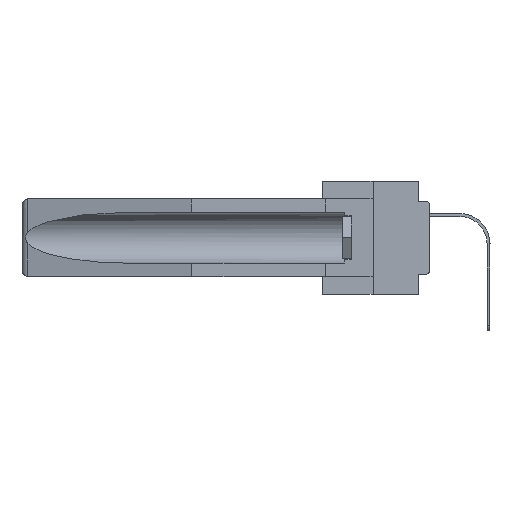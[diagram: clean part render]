
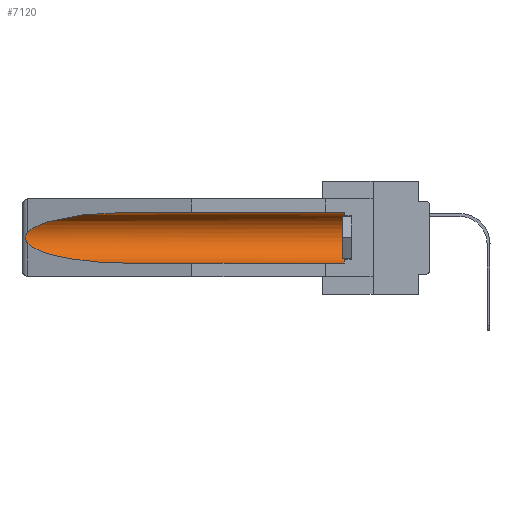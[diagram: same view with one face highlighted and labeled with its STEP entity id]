
A CAD part, left-side view. The second image highlights one B-rep face of the part: STEP entity #7120.
In plain terms, the highlighted cylindrical face has radius 2.857 mm (diameter 5.715 mm), a partial arc.
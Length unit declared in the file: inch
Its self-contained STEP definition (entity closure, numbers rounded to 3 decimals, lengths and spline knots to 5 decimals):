
#655 = ORIENTED_EDGE ( 'NONE', *, *, #25167, .F. ) ;
#1050 = CARTESIAN_POINT ( 'NONE',  ( 0.155, -0.30754, -0.284 ) ) ;
#1135 = ORIENTED_EDGE ( 'NONE', *, *, #18949, .T. ) ;
#1339 = LINE ( 'NONE', #1050, #6157 ) ;
#2214 = CARTESIAN_POINT ( 'NONE',  ( 0.26537, 1.52718, -0.19328 ) ) ;
#2487 = CARTESIAN_POINT ( 'NONE',  ( 0.26537, 1.52718, -0.19328 ) ) ;
#3384 = VERTEX_POINT ( 'NONE', #7157 ) ;
#4302 = CARTESIAN_POINT ( 'NONE',  ( 0.155, 1.07973, -0.284 ) ) ;
#4368 =( BOUNDED_CURVE ( )  B_SPLINE_CURVE ( 3, ( #22497, #22637, #20233, #8816 ),
 .UNSPECIFIED., .F., .F. ) 
 B_SPLINE_CURVE_WITH_KNOTS ( ( 4, 4 ),
 ( 4.71239, 6.08839 ),
 .UNSPECIFIED. ) 
 CURVE ( )  GEOMETRIC_REPRESENTATION_ITEM ( )  RATIONAL_B_SPLINE_CURVE ( ( 1., 0.848, 0.848, 1. ) ) 
 REPRESENTATION_ITEM ( '' )  );
#4454 = CARTESIAN_POINT ( 'NONE',  ( 0.26654, 1.53092, -0.15636 ) ) ;
#5358 = DIRECTION ( 'NONE',  ( 0., -1., 0. ) ) ;
#5659 = DIRECTION ( 'NONE',  ( 0., 0., 1. ) ) ;
#5753 = CARTESIAN_POINT ( 'NONE',  ( 0.25451, 1.48313, -0.24835 ) ) ;
#6157 = VECTOR ( 'NONE', #10702, 39.37008 ) ;
#6313 = CIRCLE ( 'NONE', #12603, 0.1125 ) ;
#6398 = CARTESIAN_POINT ( 'NONE',  ( 0.26537, 1.52718, -0.14972 ) ) ;
#6467 = VERTEX_POINT ( 'NONE', #2214 ) ;
#7002 = CARTESIAN_POINT ( 'NONE',  ( 0.26597, 1.52961, -0.15275 ) ) ;
#7120 = ADVANCED_FACE ( 'NONE', ( #10876 ), #11166, .F. ) ;
#7157 = CARTESIAN_POINT ( 'NONE',  ( 0.155, 1.07973, -0.059 ) ) ;
#7757 = EDGE_CURVE ( 'NONE', #17852, #29393, #6313, .T. ) ;
#8816 = CARTESIAN_POINT ( 'NONE',  ( 0.26537, 1.52718, -0.14972 ) ) ;
#9173 = VERTEX_POINT ( 'NONE', #6398 ) ;
#9777 = VERTEX_POINT ( 'NONE', #4302 ) ;
#10536 = EDGE_CURVE ( 'NONE', #29393, #3384, #24402, .T. ) ;
#10702 = DIRECTION ( 'NONE',  ( 0., 1., 0. ) ) ;
#10876 = FACE_OUTER_BOUND ( 'NONE', #13309, .T. ) ;
#11166 = CYLINDRICAL_SURFACE ( 'NONE', #19737, 0.1125 ) ;
#11267 = CARTESIAN_POINT ( 'NONE',  ( 0.26597, 1.5296, -0.19026 ) ) ;
#11540 = CARTESIAN_POINT ( 'NONE',  ( 0.2673, 1.5327, -0.16383 ) ) ;
#12603 = AXIS2_PLACEMENT_3D ( 'NONE', #19378, #5358, #5659 ) ;
#12727 = CARTESIAN_POINT ( 'NONE',  ( 0.21114, 1.30732, -0.284 ) ) ;
#12954 = CARTESIAN_POINT ( 'NONE',  ( 0.155, -0.30754, -0.059 ) ) ;
#13109 = B_SPLINE_CURVE_WITH_KNOTS ( 'NONE', 3,
 ( #18622, #7002, #4454, #11540, #18177, #23108, #27356, #29472, #11267, #2487 ),
 .UNSPECIFIED., .F., .F.,
 ( 4, 2, 2, 2, 4 ),
 ( 0., 0.00029, 0.00058, 0.00087, 0.00117 ),
 .UNSPECIFIED. ) ;
#13309 = EDGE_LOOP ( 'NONE', ( #1135, #24173, #13916, #655, #18756, #29010 ) ) ;
#13916 = ORIENTED_EDGE ( 'NONE', *, *, #20486, .T. ) ;
#17683 = CARTESIAN_POINT ( 'NONE',  ( 0.26537, 1.52718, -0.19328 ) ) ;
#17852 = VERTEX_POINT ( 'NONE', #20982 ) ;
#18177 = CARTESIAN_POINT ( 'NONE',  ( 0.2675, 1.53308, -0.16763 ) ) ;
#18622 = CARTESIAN_POINT ( 'NONE',  ( 0.26537, 1.52718, -0.14972 ) ) ;
#18756 = ORIENTED_EDGE ( 'NONE', *, *, #7757, .T. ) ;
#18949 = EDGE_CURVE ( 'NONE', #3384, #9173, #4368, .T. ) ;
#19170 = CARTESIAN_POINT ( 'NONE',  ( 0.155, 0.126, -0.059 ) ) ;
#19378 = CARTESIAN_POINT ( 'NONE',  ( 0.155, 0.126, -0.1715 ) ) ;
#19421 = VECTOR ( 'NONE', #22117, 39.37008 ) ;
#19737 = AXIS2_PLACEMENT_3D ( 'NONE', #20333, #29091, #26829 ) ;
#20233 = CARTESIAN_POINT ( 'NONE',  ( 0.25451, 1.48313, -0.09465 ) ) ;
#20333 = CARTESIAN_POINT ( 'NONE',  ( 0.155, -0.30754, -0.1715 ) ) ;
#20486 = EDGE_CURVE ( 'NONE', #6467, #9777, #24182, .T. ) ;
#20982 = CARTESIAN_POINT ( 'NONE',  ( 0.155, 0.126, -0.284 ) ) ;
#22117 = DIRECTION ( 'NONE',  ( 0., 1., 0. ) ) ;
#22497 = CARTESIAN_POINT ( 'NONE',  ( 0.155, 1.07973, -0.059 ) ) ;
#22637 = CARTESIAN_POINT ( 'NONE',  ( 0.21114, 1.30732, -0.059 ) ) ;
#23108 = CARTESIAN_POINT ( 'NONE',  ( 0.2675, 1.53308, -0.17534 ) ) ;
#23851 = CARTESIAN_POINT ( 'NONE',  ( 0.155, 1.07973, -0.284 ) ) ;
#23991 = EDGE_CURVE ( 'NONE', #9173, #6467, #13109, .T. ) ;
#24173 = ORIENTED_EDGE ( 'NONE', *, *, #23991, .T. ) ;
#24182 =( BOUNDED_CURVE ( )  B_SPLINE_CURVE ( 3, ( #17683, #5753, #12727, #23851 ),
 .UNSPECIFIED., .F., .F. ) 
 B_SPLINE_CURVE_WITH_KNOTS ( ( 4, 4 ),
 ( 0.1948, 1.5708 ),
 .UNSPECIFIED. ) 
 CURVE ( )  GEOMETRIC_REPRESENTATION_ITEM ( )  RATIONAL_B_SPLINE_CURVE ( ( 1., 0.848, 0.848, 1. ) ) 
 REPRESENTATION_ITEM ( '' )  );
#24402 = LINE ( 'NONE', #12954, #19421 ) ;
#25167 = EDGE_CURVE ( 'NONE', #17852, #9777, #1339, .T. ) ;
#26829 = DIRECTION ( 'NONE',  ( 0., 0., 1. ) ) ;
#27356 = CARTESIAN_POINT ( 'NONE',  ( 0.2673, 1.53269, -0.17917 ) ) ;
#29010 = ORIENTED_EDGE ( 'NONE', *, *, #10536, .T. ) ;
#29091 = DIRECTION ( 'NONE',  ( 0., 1., 0. ) ) ;
#29393 = VERTEX_POINT ( 'NONE', #19170 ) ;
#29472 = CARTESIAN_POINT ( 'NONE',  ( 0.26655, 1.53094, -0.18657 ) ) ;
